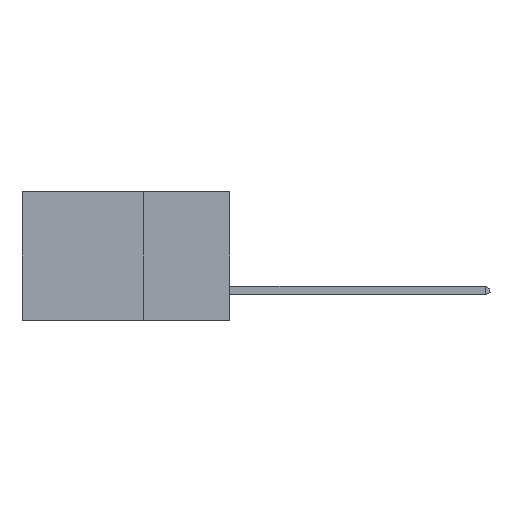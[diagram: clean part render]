
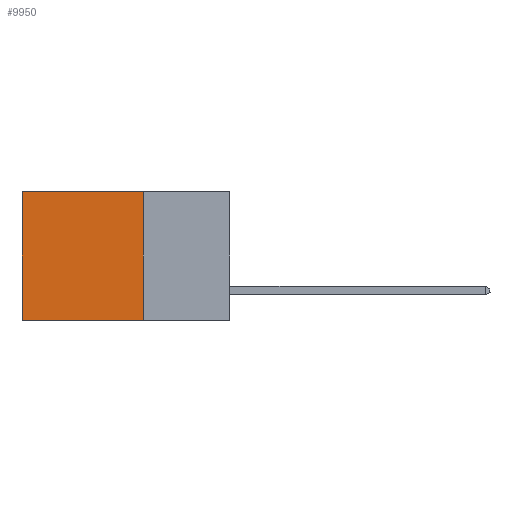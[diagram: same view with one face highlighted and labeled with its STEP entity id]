
A CAD part, left-side view. The second image highlights one B-rep face of the part: STEP entity #9950.
In plain terms, the highlighted planar face has unit normal (-1, 0, 0).
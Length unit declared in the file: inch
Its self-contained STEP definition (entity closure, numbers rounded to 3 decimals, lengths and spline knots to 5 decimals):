
#340 = LINE ( 'NONE', #9994, #11439 ) ;
#348 = DIRECTION ( 'NONE',  ( 0., 0., -1. ) ) ;
#351 = VERTEX_POINT ( 'NONE', #10870 ) ;
#383 = LINE ( 'NONE', #2826, #10377 ) ;
#1734 = ORIENTED_EDGE ( 'NONE', *, *, #5224, .T. ) ;
#2739 = ORIENTED_EDGE ( 'NONE', *, *, #5472, .T. ) ;
#2783 = CARTESIAN_POINT ( 'NONE',  ( 0.298, 0.25, -0.37 ) ) ;
#2826 = CARTESIAN_POINT ( 'NONE',  ( 0.298, 0.6, 0. ) ) ;
#3155 = DIRECTION ( 'NONE',  ( 0., 1., 0. ) ) ;
#3172 = CARTESIAN_POINT ( 'NONE',  ( 0.298, 0.25, 0. ) ) ;
#3986 = CARTESIAN_POINT ( 'NONE',  ( 0.298, 0.25, 0. ) ) ;
#4691 = VERTEX_POINT ( 'NONE', #2783 ) ;
#5015 = VECTOR ( 'NONE', #3155, 39.37008 ) ;
#5202 = FACE_OUTER_BOUND ( 'NONE', #8383, .T. ) ;
#5206 = CARTESIAN_POINT ( 'NONE',  ( 0.298, 0.25, -0.37 ) ) ;
#5224 = EDGE_CURVE ( 'NONE', #5839, #8345, #383, .T. ) ;
#5472 = EDGE_CURVE ( 'NONE', #351, #5839, #12292, .T. ) ;
#5839 = VERTEX_POINT ( 'NONE', #10840 ) ;
#6160 = ORIENTED_EDGE ( 'NONE', *, *, #11931, .F. ) ;
#6418 = CARTESIAN_POINT ( 'NONE',  ( 0.298, 0.6, -0.37 ) ) ;
#6816 = DIRECTION ( 'NONE',  ( 1., 0., 0. ) ) ;
#8345 = VERTEX_POINT ( 'NONE', #6418 ) ;
#8383 = EDGE_LOOP ( 'NONE', ( #1734, #12397, #6160, #2739 ) ) ;
#9628 = DIRECTION ( 'NONE',  ( 0., 0., -1. ) ) ;
#9760 = PLANE ( 'NONE',  #12178 ) ;
#9934 = VECTOR ( 'NONE', #10958, 39.37008 ) ;
#9950 = ADVANCED_FACE ( 'NONE', ( #5202 ), #9760, .F. ) ;
#9994 = CARTESIAN_POINT ( 'NONE',  ( 0.298, 0.25, 0. ) ) ;
#10377 = VECTOR ( 'NONE', #9628, 39.37008 ) ;
#10747 = DIRECTION ( 'NONE',  ( 0., 0., -1. ) ) ;
#10840 = CARTESIAN_POINT ( 'NONE',  ( 0.298, 0.6, 0. ) ) ;
#10870 = CARTESIAN_POINT ( 'NONE',  ( 0.298, 0.25, 0. ) ) ;
#10958 = DIRECTION ( 'NONE',  ( 0., 1., 0. ) ) ;
#11106 = LINE ( 'NONE', #5206, #5015 ) ;
#11439 = VECTOR ( 'NONE', #348, 39.37008 ) ;
#11931 = EDGE_CURVE ( 'NONE', #351, #4691, #340, .T. ) ;
#12178 = AXIS2_PLACEMENT_3D ( 'NONE', #3986, #6816, #10747 ) ;
#12292 = LINE ( 'NONE', #3172, #9934 ) ;
#12397 = ORIENTED_EDGE ( 'NONE', *, *, #12485, .F. ) ;
#12485 = EDGE_CURVE ( 'NONE', #4691, #8345, #11106, .T. ) ;
